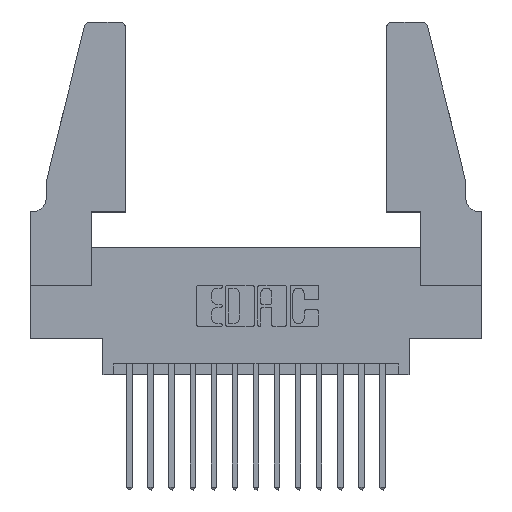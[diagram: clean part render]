
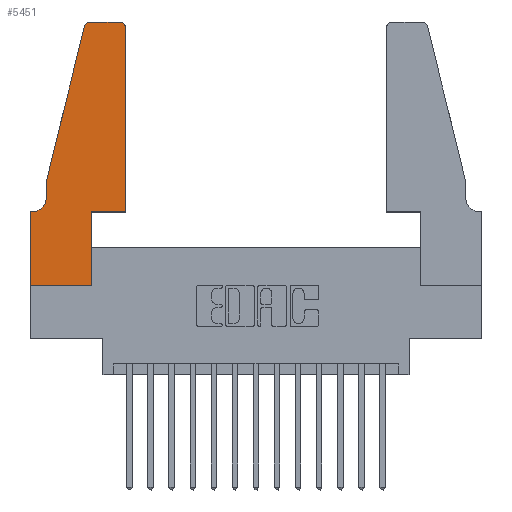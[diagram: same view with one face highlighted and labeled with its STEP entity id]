
A CAD part, top view. The second image highlights one B-rep face of the part: STEP entity #5451.
In plain terms, the highlighted planar face has unit normal (0, 0, 1).
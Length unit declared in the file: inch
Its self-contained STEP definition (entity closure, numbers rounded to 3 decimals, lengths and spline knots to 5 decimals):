
#60 = CARTESIAN_POINT ( 'NONE',  ( 0.4505, 1.22, 0.37 ) ) ;
#307 = EDGE_CURVE ( 'NONE', #5372, #11183, #13624, .T. ) ;
#427 = LINE ( 'NONE', #13888, #13546 ) ;
#465 = CARTESIAN_POINT ( 'NONE',  ( 0.2865, 0.35, 0.37 ) ) ;
#547 = LINE ( 'NONE', #16183, #6284 ) ;
#698 = VERTEX_POINT ( 'NONE', #60 ) ;
#851 = CARTESIAN_POINT ( 'NONE',  ( 0.0755, 0.35, 0.37 ) ) ;
#977 = DIRECTION ( 'NONE',  ( -1., 0., 0. ) ) ;
#1073 = VERTEX_POINT ( 'NONE', #465 ) ;
#1083 = AXIS2_PLACEMENT_3D ( 'NONE', #15438, #1677, #10611 ) ;
#1330 = DIRECTION ( 'NONE',  ( 1., 0., 0. ) ) ;
#1494 = DIRECTION ( 'NONE',  ( 0., 0., 1. ) ) ;
#1500 = CARTESIAN_POINT ( 'NONE',  ( 0.284, 1.22, 0.37 ) ) ;
#1677 = DIRECTION ( 'NONE',  ( 0., 0., 1. ) ) ;
#1680 = EDGE_CURVE ( 'NONE', #5109, #4405, #13573, .T. ) ;
#1772 = ORIENTED_EDGE ( 'NONE', *, *, #11211, .T. ) ;
#2138 = DIRECTION ( 'NONE',  ( 0., 0., -1. ) ) ;
#2620 = EDGE_CURVE ( 'NONE', #11183, #5898, #427, .T. ) ;
#3025 = CARTESIAN_POINT ( 'NONE',  ( 0.4205, 1.25, 0.37 ) ) ;
#3476 = CARTESIAN_POINT ( 'NONE',  ( 0., 0., 0.37 ) ) ;
#3623 = CARTESIAN_POINT ( 'NONE',  ( 0.4205, 1.22, 0.37 ) ) ;
#3831 = ORIENTED_EDGE ( 'NONE', *, *, #10097, .T. ) ;
#4224 = VECTOR ( 'NONE', #14634, 39.37008 ) ;
#4277 = LINE ( 'NONE', #6533, #14216 ) ;
#4405 = VERTEX_POINT ( 'NONE', #4773 ) ;
#4543 = LINE ( 'NONE', #12376, #7124 ) ;
#4658 = ORIENTED_EDGE ( 'NONE', *, *, #11777, .T. ) ;
#4767 = VERTEX_POINT ( 'NONE', #5431 ) ;
#4773 = CARTESIAN_POINT ( 'NONE',  ( 0.0055, 0.35, 0.37 ) ) ;
#4948 = DIRECTION ( 'NONE',  ( 1., 0., 0. ) ) ;
#5074 = ORIENTED_EDGE ( 'NONE', *, *, #6766, .T. ) ;
#5109 = VERTEX_POINT ( 'NONE', #9875 ) ;
#5144 = ORIENTED_EDGE ( 'NONE', *, *, #10249, .T. ) ;
#5372 = VERTEX_POINT ( 'NONE', #14131 ) ;
#5431 = CARTESIAN_POINT ( 'NONE',  ( 0., 0.35, 0.37 ) ) ;
#5451 = ADVANCED_FACE ( 'NONE', ( #11124 ), #15494, .T. ) ;
#5519 = ORIENTED_EDGE ( 'NONE', *, *, #12380, .T. ) ;
#5898 = VERTEX_POINT ( 'NONE', #13951 ) ;
#6143 = VECTOR ( 'NONE', #11950, 39.37008 ) ;
#6284 = VECTOR ( 'NONE', #11276, 39.37008 ) ;
#6524 = LINE ( 'NONE', #10735, #6143 ) ;
#6533 = CARTESIAN_POINT ( 'NONE',  ( 0.0755, 0.5, 0.37 ) ) ;
#6676 = ORIENTED_EDGE ( 'NONE', *, *, #307, .T. ) ;
#6766 = EDGE_CURVE ( 'NONE', #7370, #698, #11445, .T. ) ;
#6951 = ORIENTED_EDGE ( 'NONE', *, *, #9391, .T. ) ;
#6969 = DIRECTION ( 'NONE',  ( 0., -1., 0. ) ) ;
#7124 = VECTOR ( 'NONE', #14848, 39.37008 ) ;
#7239 = CARTESIAN_POINT ( 'NONE',  ( 0.2605, 1.25, 0.37 ) ) ;
#7262 = ORIENTED_EDGE ( 'NONE', *, *, #15970, .T. ) ;
#7370 = VERTEX_POINT ( 'NONE', #12991 ) ;
#8131 = CARTESIAN_POINT ( 'NONE',  ( 0.4505, 0.35, 0.37 ) ) ;
#8625 = EDGE_CURVE ( 'NONE', #4767, #10166, #6524, .T. ) ;
#9126 = ORIENTED_EDGE ( 'NONE', *, *, #8625, .T. ) ;
#9391 = EDGE_CURVE ( 'NONE', #10166, #13444, #15023, .T. ) ;
#9565 = CARTESIAN_POINT ( 'NONE',  ( 0.2865, 0., 0.37 ) ) ;
#9813 = CARTESIAN_POINT ( 'NONE',  ( 0.0055, 0.42, 0.37 ) ) ;
#9875 = CARTESIAN_POINT ( 'NONE',  ( 0.0755, 0.42, 0.37 ) ) ;
#10012 = LINE ( 'NONE', #851, #13641 ) ;
#10097 = EDGE_CURVE ( 'NONE', #1073, #7370, #547, .T. ) ;
#10166 = VERTEX_POINT ( 'NONE', #13844 ) ;
#10249 = EDGE_CURVE ( 'NONE', #5898, #5109, #4277, .T. ) ;
#10258 = DIRECTION ( 'NONE',  ( -0.239, -0.971, 0. ) ) ;
#10484 = AXIS2_PLACEMENT_3D ( 'NONE', #3623, #12394, #4948 ) ;
#10524 = LINE ( 'NONE', #7239, #4224 ) ;
#10611 = DIRECTION ( 'NONE',  ( 1., 0., 0. ) ) ;
#10634 = EDGE_LOOP ( 'NONE', ( #7262, #6676, #16049, #5144, #13318, #1772, #9126, #6951, #5519, #3831, #5074, #4658 ) ) ;
#10652 = CIRCLE ( 'NONE', #10484, 0.03 ) ;
#10735 = CARTESIAN_POINT ( 'NONE',  ( 0., 0., 0.37 ) ) ;
#11031 = DIRECTION ( 'NONE',  ( -1., 0., 0. ) ) ;
#11083 = VECTOR ( 'NONE', #11834, 39.37008 ) ;
#11124 = FACE_OUTER_BOUND ( 'NONE', #10634, .T. ) ;
#11127 = CARTESIAN_POINT ( 'NONE',  ( 0.25487, 1.22718, 0.37 ) ) ;
#11183 = VERTEX_POINT ( 'NONE', #11127 ) ;
#11211 = EDGE_CURVE ( 'NONE', #4405, #4767, #10012, .T. ) ;
#11276 = DIRECTION ( 'NONE',  ( 1., 0., 0. ) ) ;
#11368 = VECTOR ( 'NONE', #13498, 39.37008 ) ;
#11445 = LINE ( 'NONE', #8131, #11083 ) ;
#11468 = AXIS2_PLACEMENT_3D ( 'NONE', #9813, #2138, #11031 ) ;
#11777 = EDGE_CURVE ( 'NONE', #698, #15799, #10652, .T. ) ;
#11834 = DIRECTION ( 'NONE',  ( 0., 1., 0. ) ) ;
#11874 = AXIS2_PLACEMENT_3D ( 'NONE', #1500, #1494, #1330 ) ;
#11950 = DIRECTION ( 'NONE',  ( 0., -1., 0. ) ) ;
#12376 = CARTESIAN_POINT ( 'NONE',  ( 0.2865, 0.35, 0.37 ) ) ;
#12380 = EDGE_CURVE ( 'NONE', #13444, #1073, #4543, .T. ) ;
#12394 = DIRECTION ( 'NONE',  ( 0., 0., 1. ) ) ;
#12991 = CARTESIAN_POINT ( 'NONE',  ( 0.4505, 0.35, 0.37 ) ) ;
#13318 = ORIENTED_EDGE ( 'NONE', *, *, #1680, .T. ) ;
#13444 = VERTEX_POINT ( 'NONE', #9565 ) ;
#13498 = DIRECTION ( 'NONE',  ( 1., 0., 0. ) ) ;
#13546 = VECTOR ( 'NONE', #10258, 39.37008 ) ;
#13573 = CIRCLE ( 'NONE', #11468, 0.07 ) ;
#13624 = CIRCLE ( 'NONE', #11874, 0.03 ) ;
#13641 = VECTOR ( 'NONE', #977, 39.37008 ) ;
#13844 = CARTESIAN_POINT ( 'NONE',  ( 0., 0., 0.37 ) ) ;
#13888 = CARTESIAN_POINT ( 'NONE',  ( 0.0755, 0.5, 0.37 ) ) ;
#13951 = CARTESIAN_POINT ( 'NONE',  ( 0.0755, 0.5, 0.37 ) ) ;
#14131 = CARTESIAN_POINT ( 'NONE',  ( 0.284, 1.25, 0.37 ) ) ;
#14216 = VECTOR ( 'NONE', #6969, 39.37008 ) ;
#14634 = DIRECTION ( 'NONE',  ( -1., 0., 0. ) ) ;
#14848 = DIRECTION ( 'NONE',  ( 0., 1., 0. ) ) ;
#15023 = LINE ( 'NONE', #3476, #11368 ) ;
#15438 = CARTESIAN_POINT ( 'NONE',  ( 0., 0.35, 0.37 ) ) ;
#15494 = PLANE ( 'NONE',  #1083 ) ;
#15799 = VERTEX_POINT ( 'NONE', #3025 ) ;
#15970 = EDGE_CURVE ( 'NONE', #15799, #5372, #10524, .T. ) ;
#16049 = ORIENTED_EDGE ( 'NONE', *, *, #2620, .T. ) ;
#16183 = CARTESIAN_POINT ( 'NONE',  ( 0.4505, 0.35, 0.37 ) ) ;
